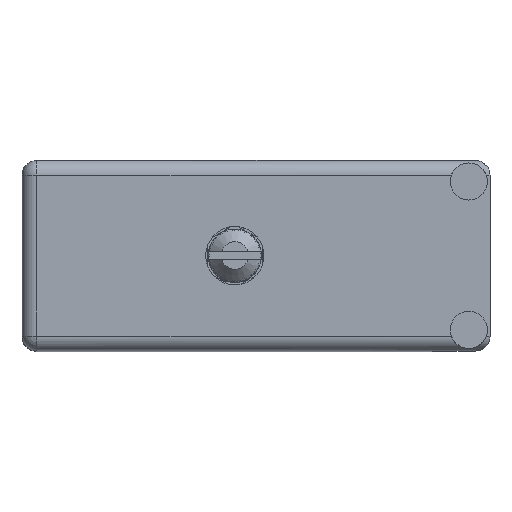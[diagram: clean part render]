
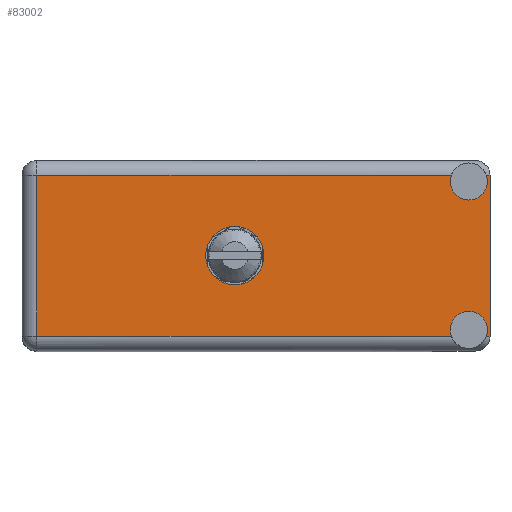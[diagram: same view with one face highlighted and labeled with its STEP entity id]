
A CAD part, top view. The second image highlights one B-rep face of the part: STEP entity #83002.
In plain terms, the highlighted face is planar.
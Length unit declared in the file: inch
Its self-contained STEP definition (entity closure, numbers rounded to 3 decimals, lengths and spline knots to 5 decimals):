
#1 = CARTESIAN_POINT ( 'NONE',  ( 2.02562, 1.566, -0.07 ) ) ;
#145 = ORIENTED_EDGE ( 'NONE', *, *, #13046, .F. ) ;
#2785 = CARTESIAN_POINT ( 'NONE',  ( 0.07, 1.566, -0.899 ) ) ;
#3902 = VERTEX_POINT ( 'NONE', #87356 ) ;
#4098 = VERTEX_POINT ( 'NONE', #69884 ) ;
#4175 = DIRECTION ( 'NONE',  ( 0., 0., 1. ) ) ;
#4749 = AXIS2_PLACEMENT_3D ( 'NONE', #40275, #83522, #4175 ) ;
#5070 = VECTOR ( 'NONE', #95851, 39.37008 ) ;
#5659 = ORIENTED_EDGE ( 'NONE', *, *, #22860, .T. ) ;
#6139 = DIRECTION ( 'NONE',  ( 0., 1., 0. ) ) ;
#7306 = CIRCLE ( 'NONE', #4749, 0.0875 ) ;
#9278 = VERTEX_POINT ( 'NONE', #56134 ) ;
#9569 = CARTESIAN_POINT ( 'NONE',  ( 2.19038, 1.566, -0.829 ) ) ;
#11025 = EDGE_CURVE ( 'NONE', #93172, #3902, #97777, .T. ) ;
#13046 = EDGE_CURVE ( 'NONE', #97562, #9278, #30609, .T. ) ;
#13182 = CARTESIAN_POINT ( 'NONE',  ( 2.108, 1.566, -0.187 ) ) ;
#14088 = VERTEX_POINT ( 'NONE', #13182 ) ;
#14702 = CARTESIAN_POINT ( 'NONE',  ( 0., 1.566, -0.899 ) ) ;
#15734 = EDGE_LOOP ( 'NONE', ( #47028, #94066, #16350, #87952, #24619, #5659, #44447, #145, #33092, #18687 ) ) ;
#15868 = EDGE_CURVE ( 'NONE', #29636, #16200, #65154, .T. ) ;
#16200 = VERTEX_POINT ( 'NONE', #32231 ) ;
#16350 = ORIENTED_EDGE ( 'NONE', *, *, #100464, .F. ) ;
#18687 = ORIENTED_EDGE ( 'NONE', *, *, #11025, .T. ) ;
#18783 = DIRECTION ( 'NONE',  ( 1., 0., 0. ) ) ;
#19013 = CARTESIAN_POINT ( 'NONE',  ( 2.208, 1.566, -0.07 ) ) ;
#19188 = VECTOR ( 'NONE', #110758, 39.37008 ) ;
#20926 = CARTESIAN_POINT ( 'NONE',  ( 0.07, 1.566, -0.829 ) ) ;
#22860 = EDGE_CURVE ( 'NONE', #70265, #113746, #67678, .T. ) ;
#23847 = CARTESIAN_POINT ( 'NONE',  ( 0., 1.566, -0.829 ) ) ;
#23939 = EDGE_CURVE ( 'NONE', #4098, #82679, #32716, .T. ) ;
#24619 = ORIENTED_EDGE ( 'NONE', *, *, #27805, .F. ) ;
#27588 = DIRECTION ( 'NONE',  ( 1., 0., 0. ) ) ;
#27805 = EDGE_CURVE ( 'NONE', #70265, #82679, #93379, .T. ) ;
#28590 = CARTESIAN_POINT ( 'NONE',  ( 2.108, 1.566, -0.7995 ) ) ;
#29636 = VERTEX_POINT ( 'NONE', #69090 ) ;
#30609 = CIRCLE ( 'NONE', #60491, 0.0875 ) ;
#32231 = CARTESIAN_POINT ( 'NONE',  ( 1.004, 1.566, -0.312 ) ) ;
#32369 = CARTESIAN_POINT ( 'NONE',  ( 1.004, 1.566, -0.4495 ) ) ;
#32716 = LINE ( 'NONE', #72879, #67560 ) ;
#33092 = ORIENTED_EDGE ( 'NONE', *, *, #33409, .T. ) ;
#33409 = EDGE_CURVE ( 'NONE', #97562, #93172, #93016, .T. ) ;
#38443 = FACE_BOUND ( 'NONE', #50103, .T. ) ;
#40275 = CARTESIAN_POINT ( 'NONE',  ( 2.108, 1.566, -0.0995 ) ) ;
#41537 = CARTESIAN_POINT ( 'NONE',  ( 2.208, 1.566, -0.829 ) ) ;
#41921 = PLANE ( 'NONE',  #93377 ) ;
#42087 = EDGE_CURVE ( 'NONE', #14088, #98818, #94533, .T. ) ;
#42122 = LINE ( 'NONE', #19013, #82308 ) ;
#42989 = ORIENTED_EDGE ( 'NONE', *, *, #85738, .F. ) ;
#43009 = DIRECTION ( 'NONE',  ( 0., 0., 1. ) ) ;
#43560 = CARTESIAN_POINT ( 'NONE',  ( 1.004, 1.566, -0.4495 ) ) ;
#44447 = ORIENTED_EDGE ( 'NONE', *, *, #66136, .F. ) ;
#47028 = ORIENTED_EDGE ( 'NONE', *, *, #106096, .T. ) ;
#48408 = CARTESIAN_POINT ( 'NONE',  ( 0., 1.566, -0.829 ) ) ;
#50103 = EDGE_LOOP ( 'NONE', ( #42989, #95416 ) ) ;
#50807 = CARTESIAN_POINT ( 'NONE',  ( 2.108, 1.566, -0.7995 ) ) ;
#54730 = DIRECTION ( 'NONE',  ( 0., 0., 1. ) ) ;
#56134 = CARTESIAN_POINT ( 'NONE',  ( 2.108, 1.566, -0.712 ) ) ;
#58546 = DIRECTION ( 'NONE',  ( 0., 0., 1. ) ) ;
#59172 = AXIS2_PLACEMENT_3D ( 'NONE', #28590, #108099, #54730 ) ;
#60491 = AXIS2_PLACEMENT_3D ( 'NONE', #50807, #103724, #86148 ) ;
#62406 = CARTESIAN_POINT ( 'NONE',  ( 2.02562, 1.566, -0.829 ) ) ;
#62821 = VECTOR ( 'NONE', #43009, 39.37008 ) ;
#65154 = CIRCLE ( 'NONE', #81588, 0.1375 ) ;
#66136 = EDGE_CURVE ( 'NONE', #9278, #113746, #71349, .T. ) ;
#66193 = DIRECTION ( 'NONE',  ( 0., 1., 0. ) ) ;
#67560 = VECTOR ( 'NONE', #18783, 39.37008 ) ;
#67678 = LINE ( 'NONE', #23847, #5070 ) ;
#69090 = CARTESIAN_POINT ( 'NONE',  ( 1.004, 1.566, -0.587 ) ) ;
#69884 = CARTESIAN_POINT ( 'NONE',  ( 2.19038, 1.566, -0.07 ) ) ;
#70265 = VERTEX_POINT ( 'NONE', #41537 ) ;
#70547 = FACE_OUTER_BOUND ( 'NONE', #15734, .T. ) ;
#71349 = CIRCLE ( 'NONE', #59172, 0.0875 ) ;
#72879 = CARTESIAN_POINT ( 'NONE',  ( 2.208, 1.566, -0.07 ) ) ;
#78650 = DIRECTION ( 'NONE',  ( 0., 0., 1. ) ) ;
#81588 = AXIS2_PLACEMENT_3D ( 'NONE', #32369, #103648, #58546 ) ;
#82308 = VECTOR ( 'NONE', #27588, 39.37008 ) ;
#82679 = VERTEX_POINT ( 'NONE', #96140 ) ;
#83002 = ADVANCED_FACE ( 'NONE', ( #38443, #70547 ), #41921, .T. ) ;
#83522 = DIRECTION ( 'NONE',  ( 0., 1., 0. ) ) ;
#85738 = EDGE_CURVE ( 'NONE', #16200, #29636, #93940, .T. ) ;
#86148 = DIRECTION ( 'NONE',  ( 0., 0., 1. ) ) ;
#87356 = CARTESIAN_POINT ( 'NONE',  ( 0.07, 1.566, -0.07 ) ) ;
#87952 = ORIENTED_EDGE ( 'NONE', *, *, #23939, .T. ) ;
#92284 = CARTESIAN_POINT ( 'NONE',  ( 2.108, 1.566, -0.0995 ) ) ;
#93016 = LINE ( 'NONE', #48408, #19188 ) ;
#93172 = VERTEX_POINT ( 'NONE', #20926 ) ;
#93377 = AXIS2_PLACEMENT_3D ( 'NONE', #14702, #6139, #104613 ) ;
#93379 = LINE ( 'NONE', #114330, #62821 ) ;
#93491 = VECTOR ( 'NONE', #108320, 39.37008 ) ;
#93940 = CIRCLE ( 'NONE', #115492, 0.1375 ) ;
#94066 = ORIENTED_EDGE ( 'NONE', *, *, #42087, .F. ) ;
#94533 = CIRCLE ( 'NONE', #109174, 0.0875 ) ;
#95416 = ORIENTED_EDGE ( 'NONE', *, *, #15868, .F. ) ;
#95851 = DIRECTION ( 'NONE',  ( -1., 0., 0. ) ) ;
#96140 = CARTESIAN_POINT ( 'NONE',  ( 2.208, 1.566, -0.07 ) ) ;
#97562 = VERTEX_POINT ( 'NONE', #62406 ) ;
#97777 = LINE ( 'NONE', #2785, #93491 ) ;
#98818 = VERTEX_POINT ( 'NONE', #1 ) ;
#100464 = EDGE_CURVE ( 'NONE', #4098, #14088, #7306, .T. ) ;
#102039 = DIRECTION ( 'NONE',  ( 0., 0., 1. ) ) ;
#103648 = DIRECTION ( 'NONE',  ( 0., 1., 0. ) ) ;
#103724 = DIRECTION ( 'NONE',  ( 0., 1., 0. ) ) ;
#104613 = DIRECTION ( 'NONE',  ( 0., 0., 1. ) ) ;
#105490 = DIRECTION ( 'NONE',  ( 0., 1., 0. ) ) ;
#106096 = EDGE_CURVE ( 'NONE', #3902, #98818, #42122, .T. ) ;
#108099 = DIRECTION ( 'NONE',  ( 0., 1., 0. ) ) ;
#108320 = DIRECTION ( 'NONE',  ( 0., 0., 1. ) ) ;
#109174 = AXIS2_PLACEMENT_3D ( 'NONE', #92284, #66193, #102039 ) ;
#110758 = DIRECTION ( 'NONE',  ( -1., 0., 0. ) ) ;
#113746 = VERTEX_POINT ( 'NONE', #9569 ) ;
#114330 = CARTESIAN_POINT ( 'NONE',  ( 2.208, 1.566, 0. ) ) ;
#115492 = AXIS2_PLACEMENT_3D ( 'NONE', #43560, #105490, #78650 ) ;
